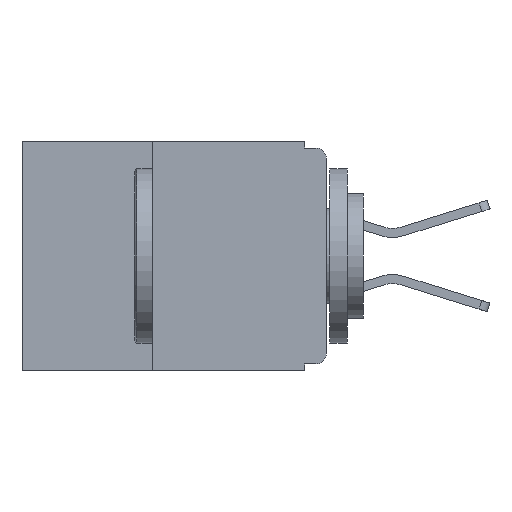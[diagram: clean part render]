
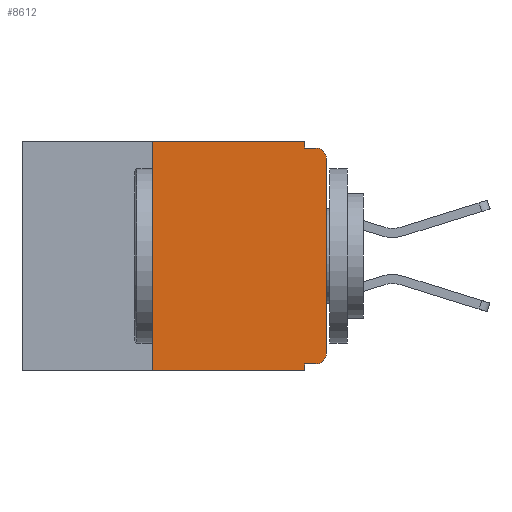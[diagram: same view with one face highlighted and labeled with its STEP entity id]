
A CAD part, left-side view. The second image highlights one B-rep face of the part: STEP entity #8612.
In plain terms, the highlighted planar face has unit normal (-1, 0, 0).
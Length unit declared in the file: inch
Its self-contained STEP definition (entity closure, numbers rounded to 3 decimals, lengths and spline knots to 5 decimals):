
#158 = EDGE_CURVE ( 'NONE', #22385, #11552, #11842, .T. ) ;
#524 = EDGE_LOOP ( 'NONE', ( #7864, #24666, #22799, #14577, #23733, #15527, #18453, #6211, #8630, #9210 ) ) ;
#809 = DIRECTION ( 'NONE',  ( -1., 0., 0. ) ) ;
#924 = VECTOR ( 'NONE', #22237, 39.37008 ) ;
#1350 = DIRECTION ( 'NONE',  ( 0., -1., 0. ) ) ;
#1373 = VERTEX_POINT ( 'NONE', #22912 ) ;
#2320 = DIRECTION ( 'NONE',  ( 0., 0., 1. ) ) ;
#2924 = EDGE_CURVE ( 'NONE', #7616, #22385, #22802, .T. ) ;
#3633 = LINE ( 'NONE', #11694, #8431 ) ;
#4527 = DIRECTION ( 'NONE',  ( -1., 0., 0. ) ) ;
#4781 = CARTESIAN_POINT ( 'NONE',  ( 0., 0.015, -0.01 ) ) ;
#4817 = CARTESIAN_POINT ( 'NONE',  ( 0., 0.437, 0. ) ) ;
#5164 = VECTOR ( 'NONE', #1350, 39.37008 ) ;
#5862 = CARTESIAN_POINT ( 'NONE',  ( 0., 0.015, -0.32 ) ) ;
#6087 = EDGE_CURVE ( 'NONE', #22506, #21970, #18740, .T. ) ;
#6211 = ORIENTED_EDGE ( 'NONE', *, *, #158, .F. ) ;
#6871 = DIRECTION ( 'NONE',  ( 0., 0., -1. ) ) ;
#6939 = LINE ( 'NONE', #14089, #924 ) ;
#7616 = VERTEX_POINT ( 'NONE', #5862 ) ;
#7666 = VERTEX_POINT ( 'NONE', #4781 ) ;
#7864 = ORIENTED_EDGE ( 'NONE', *, *, #14671, .T. ) ;
#7911 = VECTOR ( 'NONE', #14067, 39.37008 ) ;
#8431 = VECTOR ( 'NONE', #21846, 39.37008 ) ;
#8612 = ADVANCED_FACE ( 'NONE', ( #12190 ), #14963, .F. ) ;
#8630 = ORIENTED_EDGE ( 'NONE', *, *, #2924, .F. ) ;
#8697 = VECTOR ( 'NONE', #25697, 39.37008 ) ;
#9210 = ORIENTED_EDGE ( 'NONE', *, *, #21028, .T. ) ;
#10986 = CIRCLE ( 'NONE', #17508, 0.015 ) ;
#11215 = VECTOR ( 'NONE', #24132, 39.37008 ) ;
#11449 = CARTESIAN_POINT ( 'NONE',  ( 0., 0.437, 0. ) ) ;
#11552 = VERTEX_POINT ( 'NONE', #23993 ) ;
#11694 = CARTESIAN_POINT ( 'NONE',  ( 0., 0., -0.01 ) ) ;
#11842 = LINE ( 'NONE', #18867, #11215 ) ;
#12190 = FACE_OUTER_BOUND ( 'NONE', #524, .T. ) ;
#12872 = EDGE_CURVE ( 'NONE', #16555, #21504, #16559, .T. ) ;
#12925 = CARTESIAN_POINT ( 'NONE',  ( 0., 0.015, -0.025 ) ) ;
#14067 = DIRECTION ( 'NONE',  ( 0., 0., -1. ) ) ;
#14089 = CARTESIAN_POINT ( 'NONE',  ( 0., 0., 0. ) ) ;
#14102 = CARTESIAN_POINT ( 'NONE',  ( 0., 0.031, 0. ) ) ;
#14577 = ORIENTED_EDGE ( 'NONE', *, *, #6087, .F. ) ;
#14671 = EDGE_CURVE ( 'NONE', #1373, #24901, #6939, .T. ) ;
#14963 = PLANE ( 'NONE',  #24250 ) ;
#15014 = DIRECTION ( 'NONE',  ( 0., 0., -1. ) ) ;
#15527 = ORIENTED_EDGE ( 'NONE', *, *, #12872, .F. ) ;
#15565 = CARTESIAN_POINT ( 'NONE',  ( 0., 0.031, -0.01 ) ) ;
#16045 = EDGE_CURVE ( 'NONE', #24901, #7666, #10986, .T. ) ;
#16555 = VERTEX_POINT ( 'NONE', #24612 ) ;
#16559 = LINE ( 'NONE', #24572, #21356 ) ;
#16670 = CARTESIAN_POINT ( 'NONE',  ( 0., 0.015, -0.305 ) ) ;
#17201 = CARTESIAN_POINT ( 'NONE',  ( 0., 0., -0.025 ) ) ;
#17227 = CARTESIAN_POINT ( 'NONE',  ( 0., 0.031, 0. ) ) ;
#17419 = VECTOR ( 'NONE', #18737, 39.37008 ) ;
#17508 = AXIS2_PLACEMENT_3D ( 'NONE', #12925, #809, #15014 ) ;
#17521 = LINE ( 'NONE', #11449, #5164 ) ;
#18453 = ORIENTED_EDGE ( 'NONE', *, *, #23742, .T. ) ;
#18737 = DIRECTION ( 'NONE',  ( 0., 1., 0. ) ) ;
#18740 = LINE ( 'NONE', #14102, #7911 ) ;
#18743 = DIRECTION ( 'NONE',  ( 0., 0., -1. ) ) ;
#18867 = CARTESIAN_POINT ( 'NONE',  ( 0., 0.031, -0.33 ) ) ;
#18941 = CARTESIAN_POINT ( 'NONE',  ( 0., 0.031, -0.32 ) ) ;
#19055 = DIRECTION ( 'NONE',  ( 1., 0., 0. ) ) ;
#20656 = CARTESIAN_POINT ( 'NONE',  ( 0., 0.25, 0. ) ) ;
#21028 = EDGE_CURVE ( 'NONE', #7616, #1373, #21538, .T. ) ;
#21140 = CARTESIAN_POINT ( 'NONE',  ( 0., 0., -0.32 ) ) ;
#21356 = VECTOR ( 'NONE', #2320, 39.37008 ) ;
#21504 = VERTEX_POINT ( 'NONE', #20656 ) ;
#21538 = CIRCLE ( 'NONE', #22029, 0.015 ) ;
#21846 = DIRECTION ( 'NONE',  ( 0., -1., 0. ) ) ;
#21970 = VERTEX_POINT ( 'NONE', #15565 ) ;
#22029 = AXIS2_PLACEMENT_3D ( 'NONE', #16670, #4527, #18743 ) ;
#22237 = DIRECTION ( 'NONE',  ( 0., 0., 1. ) ) ;
#22385 = VERTEX_POINT ( 'NONE', #18941 ) ;
#22506 = VERTEX_POINT ( 'NONE', #17227 ) ;
#22647 = EDGE_CURVE ( 'NONE', #21970, #7666, #3633, .T. ) ;
#22799 = ORIENTED_EDGE ( 'NONE', *, *, #22647, .F. ) ;
#22802 = LINE ( 'NONE', #21140, #17419 ) ;
#22912 = CARTESIAN_POINT ( 'NONE',  ( 0., 0., -0.305 ) ) ;
#23691 = CARTESIAN_POINT ( 'NONE',  ( 0., 0.437, -0.33 ) ) ;
#23733 = ORIENTED_EDGE ( 'NONE', *, *, #24378, .F. ) ;
#23742 = EDGE_CURVE ( 'NONE', #16555, #11552, #24816, .T. ) ;
#23993 = CARTESIAN_POINT ( 'NONE',  ( 0., 0.031, -0.33 ) ) ;
#24132 = DIRECTION ( 'NONE',  ( 0., 0., -1. ) ) ;
#24250 = AXIS2_PLACEMENT_3D ( 'NONE', #4817, #19055, #6871 ) ;
#24378 = EDGE_CURVE ( 'NONE', #21504, #22506, #17521, .T. ) ;
#24572 = CARTESIAN_POINT ( 'NONE',  ( 0., 0.25, -0.33 ) ) ;
#24612 = CARTESIAN_POINT ( 'NONE',  ( 0., 0.25, -0.33 ) ) ;
#24666 = ORIENTED_EDGE ( 'NONE', *, *, #16045, .T. ) ;
#24816 = LINE ( 'NONE', #23691, #8697 ) ;
#24901 = VERTEX_POINT ( 'NONE', #17201 ) ;
#25697 = DIRECTION ( 'NONE',  ( 0., -1., 0. ) ) ;
